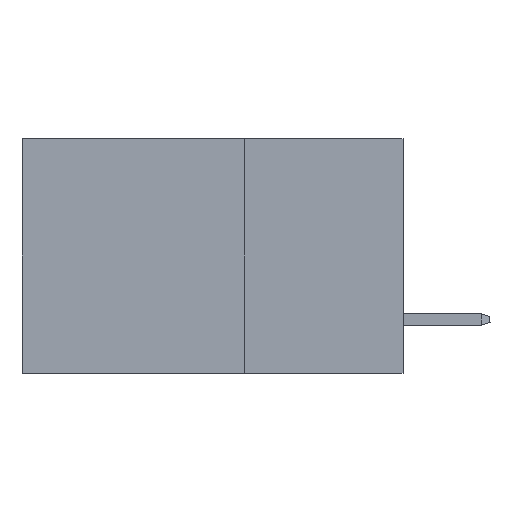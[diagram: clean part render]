
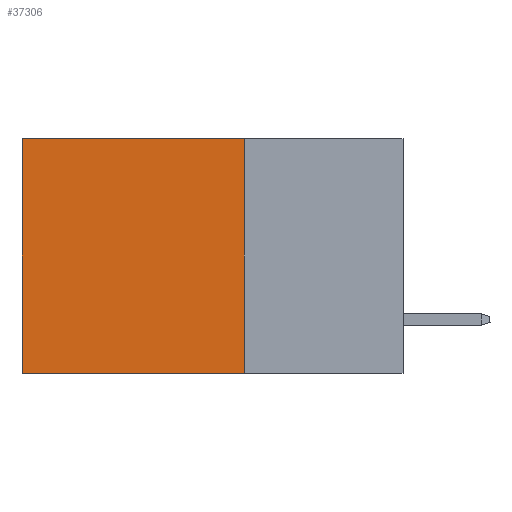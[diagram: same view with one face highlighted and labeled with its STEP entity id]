
A CAD part, left-side view. The second image highlights one B-rep face of the part: STEP entity #37306.
In plain terms, the highlighted planar face has unit normal (-1, 0, 0).
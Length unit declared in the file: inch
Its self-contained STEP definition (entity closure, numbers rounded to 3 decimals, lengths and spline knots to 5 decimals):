
#1685 = ORIENTED_EDGE ( 'NONE', *, *, #34524, .T. ) ;
#1937 = VECTOR ( 'NONE', #16282, 39.37008 ) ;
#2041 = EDGE_CURVE ( 'NONE', #44117, #25204, #27622, .T. ) ;
#3375 = EDGE_CURVE ( 'NONE', #36943, #44117, #18227, .T. ) ;
#3695 = CARTESIAN_POINT ( 'NONE',  ( 0.2875, 0.25, 0. ) ) ;
#3984 = ORIENTED_EDGE ( 'NONE', *, *, #41462, .T. ) ;
#7306 = CARTESIAN_POINT ( 'NONE',  ( 0.2875, 0.25, -0.37 ) ) ;
#9483 = LINE ( 'NONE', #41124, #1937 ) ;
#10324 = ORIENTED_EDGE ( 'NONE', *, *, #3375, .F. ) ;
#11460 = DIRECTION ( 'NONE',  ( 0., 0., -1. ) ) ;
#14309 = DIRECTION ( 'NONE',  ( 0., 1., 0. ) ) ;
#16282 = DIRECTION ( 'NONE',  ( 0., 0., -1. ) ) ;
#16776 = VERTEX_POINT ( 'NONE', #27818 ) ;
#17470 = LINE ( 'NONE', #44594, #38455 ) ;
#18227 = LINE ( 'NONE', #20924, #36978 ) ;
#20862 = FACE_OUTER_BOUND ( 'NONE', #30363, .T. ) ;
#20924 = CARTESIAN_POINT ( 'NONE',  ( 0.2875, 0.25, 0. ) ) ;
#24076 = CARTESIAN_POINT ( 'NONE',  ( 0.2875, 0.25, 0. ) ) ;
#25204 = VERTEX_POINT ( 'NONE', #41094 ) ;
#26264 = CARTESIAN_POINT ( 'NONE',  ( 0.2875, 0.25, -0.37 ) ) ;
#27622 = LINE ( 'NONE', #7306, #32487 ) ;
#27818 = CARTESIAN_POINT ( 'NONE',  ( 0.2875, 0.6, 0. ) ) ;
#28154 = ORIENTED_EDGE ( 'NONE', *, *, #2041, .F. ) ;
#29916 = AXIS2_PLACEMENT_3D ( 'NONE', #3695, #40788, #31250 ) ;
#30363 = EDGE_LOOP ( 'NONE', ( #3984, #28154, #10324, #1685 ) ) ;
#31250 = DIRECTION ( 'NONE',  ( 0., 0., -1. ) ) ;
#32487 = VECTOR ( 'NONE', #38285, 39.37008 ) ;
#34524 = EDGE_CURVE ( 'NONE', #36943, #16776, #17470, .T. ) ;
#34664 = PLANE ( 'NONE',  #29916 ) ;
#36943 = VERTEX_POINT ( 'NONE', #24076 ) ;
#36978 = VECTOR ( 'NONE', #11460, 39.37008 ) ;
#37306 = ADVANCED_FACE ( 'NONE', ( #20862 ), #34664, .F. ) ;
#38285 = DIRECTION ( 'NONE',  ( 0., 1., 0. ) ) ;
#38455 = VECTOR ( 'NONE', #14309, 39.37008 ) ;
#40788 = DIRECTION ( 'NONE',  ( 1., 0., 0. ) ) ;
#41094 = CARTESIAN_POINT ( 'NONE',  ( 0.2875, 0.6, -0.37 ) ) ;
#41124 = CARTESIAN_POINT ( 'NONE',  ( 0.2875, 0.6, 0. ) ) ;
#41462 = EDGE_CURVE ( 'NONE', #16776, #25204, #9483, .T. ) ;
#44117 = VERTEX_POINT ( 'NONE', #26264 ) ;
#44594 = CARTESIAN_POINT ( 'NONE',  ( 0.2875, 0.25, 0. ) ) ;
